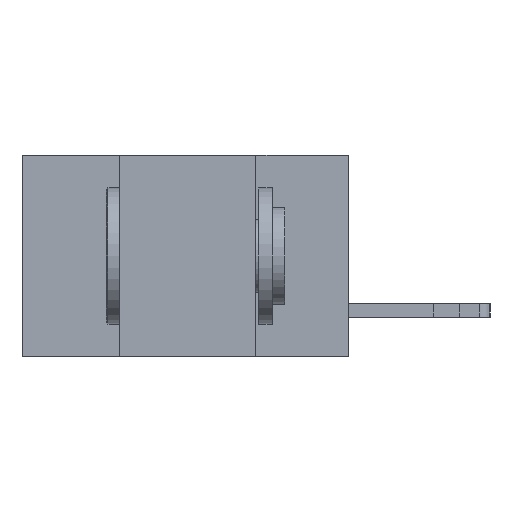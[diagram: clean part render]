
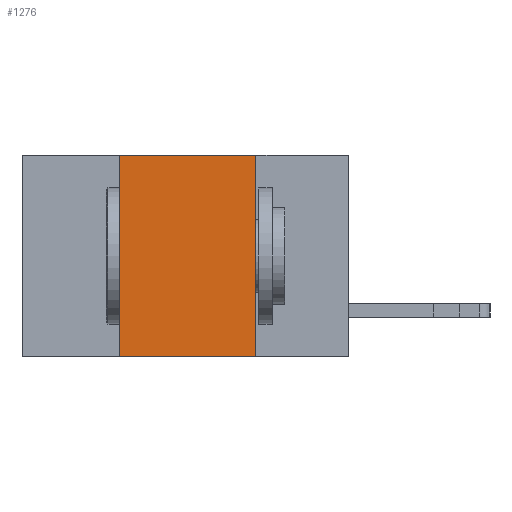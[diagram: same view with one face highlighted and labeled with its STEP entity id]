
A CAD part, left-side view. The second image highlights one B-rep face of the part: STEP entity #1276.
In plain terms, the highlighted planar face has unit normal (-1, 0, 0).
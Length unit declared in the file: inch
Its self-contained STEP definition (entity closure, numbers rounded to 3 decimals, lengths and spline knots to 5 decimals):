
#118 = VERTEX_POINT ( 'NONE', #9315 ) ;
#289 = AXIS2_PLACEMENT_3D ( 'NONE', #6685, #3954, #13660 ) ;
#449 = CARTESIAN_POINT ( 'NONE',  ( 0., 0.6, -0.37 ) ) ;
#1276 = ADVANCED_FACE ( 'NONE', ( #12917 ), #1719, .F. ) ;
#1719 = PLANE ( 'NONE',  #289 ) ;
#1886 = LINE ( 'NONE', #14626, #11189 ) ;
#1998 = CARTESIAN_POINT ( 'NONE',  ( 0., 0.6, 0. ) ) ;
#3212 = DIRECTION ( 'NONE',  ( 0., -1., 0. ) ) ;
#3954 = DIRECTION ( 'NONE',  ( 1., 0., 0. ) ) ;
#4734 = VECTOR ( 'NONE', #3212, 39.37008 ) ;
#5909 = CARTESIAN_POINT ( 'NONE',  ( 0., 0.17, -0.37 ) ) ;
#6513 = LINE ( 'NONE', #6677, #12815 ) ;
#6677 = CARTESIAN_POINT ( 'NONE',  ( 0., 0.17, 0. ) ) ;
#6685 = CARTESIAN_POINT ( 'NONE',  ( 0., 0.6, 0. ) ) ;
#6734 = EDGE_CURVE ( 'NONE', #13567, #14667, #6513, .T. ) ;
#7283 = VECTOR ( 'NONE', #8908, 39.37008 ) ;
#7651 = DIRECTION ( 'NONE',  ( 0., 0., 1. ) ) ;
#7852 = EDGE_CURVE ( 'NONE', #118, #14667, #9336, .T. ) ;
#8179 = EDGE_CURVE ( 'NONE', #14817, #13567, #14207, .T. ) ;
#8594 = CARTESIAN_POINT ( 'NONE',  ( 0., 0.42, 0. ) ) ;
#8908 = DIRECTION ( 'NONE',  ( 0., -1., 0. ) ) ;
#9315 = CARTESIAN_POINT ( 'NONE',  ( 0., 0.42, -0.37 ) ) ;
#9336 = LINE ( 'NONE', #449, #7283 ) ;
#9843 = CARTESIAN_POINT ( 'NONE',  ( 0., 0.17, 0. ) ) ;
#9898 = ORIENTED_EDGE ( 'NONE', *, *, #11788, .F. ) ;
#9955 = EDGE_LOOP ( 'NONE', ( #13151, #10451, #9898, #10995 ) ) ;
#10451 = ORIENTED_EDGE ( 'NONE', *, *, #8179, .F. ) ;
#10995 = ORIENTED_EDGE ( 'NONE', *, *, #7852, .T. ) ;
#11189 = VECTOR ( 'NONE', #7651, 39.37008 ) ;
#11788 = EDGE_CURVE ( 'NONE', #118, #14817, #1886, .T. ) ;
#12815 = VECTOR ( 'NONE', #14855, 39.37008 ) ;
#12917 = FACE_OUTER_BOUND ( 'NONE', #9955, .T. ) ;
#13151 = ORIENTED_EDGE ( 'NONE', *, *, #6734, .F. ) ;
#13567 = VERTEX_POINT ( 'NONE', #9843 ) ;
#13660 = DIRECTION ( 'NONE',  ( 0., 0., -1. ) ) ;
#14207 = LINE ( 'NONE', #1998, #4734 ) ;
#14626 = CARTESIAN_POINT ( 'NONE',  ( 0., 0.42, 0. ) ) ;
#14667 = VERTEX_POINT ( 'NONE', #5909 ) ;
#14817 = VERTEX_POINT ( 'NONE', #8594 ) ;
#14855 = DIRECTION ( 'NONE',  ( 0., 0., -1. ) ) ;
